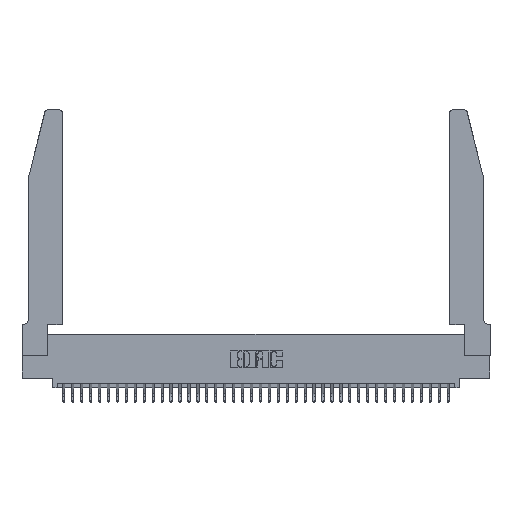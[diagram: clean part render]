
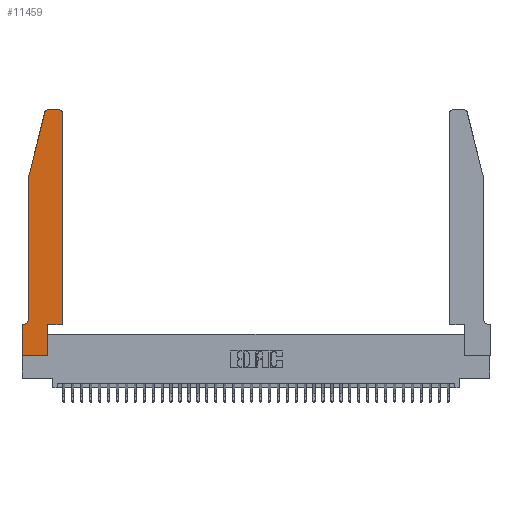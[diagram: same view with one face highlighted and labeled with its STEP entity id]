
A CAD part, top view. The second image highlights one B-rep face of the part: STEP entity #11459.
In plain terms, the highlighted planar face has unit normal (0, 0, 1).
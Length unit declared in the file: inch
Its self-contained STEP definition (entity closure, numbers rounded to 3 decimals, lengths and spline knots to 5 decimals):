
#337 = DIRECTION ( 'NONE',  ( 0., 1., 0. ) ) ;
#662 = CARTESIAN_POINT ( 'NONE',  ( 0.2865, 0.35, 0.37 ) ) ;
#986 = VECTOR ( 'NONE', #16394, 39.37008 ) ;
#1075 = VECTOR ( 'NONE', #16788, 39.37008 ) ;
#1171 = CIRCLE ( 'NONE', #2371, 0.07 ) ;
#1643 = VERTEX_POINT ( 'NONE', #33704 ) ;
#1840 = EDGE_CURVE ( 'NONE', #24150, #3727, #38521, .T. ) ;
#2062 = LINE ( 'NONE', #37913, #1075 ) ;
#2216 = VECTOR ( 'NONE', #2494, 39.37008 ) ;
#2371 = AXIS2_PLACEMENT_3D ( 'NONE', #33833, #15726, #36857 ) ;
#2494 = DIRECTION ( 'NONE',  ( 1., 0., 0. ) ) ;
#3075 = CARTESIAN_POINT ( 'NONE',  ( 0.4505, 0.35, 0.37 ) ) ;
#3687 = ORIENTED_EDGE ( 'NONE', *, *, #26643, .T. ) ;
#3727 = VERTEX_POINT ( 'NONE', #38677 ) ;
#3834 = CARTESIAN_POINT ( 'NONE',  ( 0.0755, 0.35, 0.37 ) ) ;
#4285 = VERTEX_POINT ( 'NONE', #16889 ) ;
#4536 = VERTEX_POINT ( 'NONE', #33355 ) ;
#5559 = AXIS2_PLACEMENT_3D ( 'NONE', #28609, #31632, #13505 ) ;
#5851 = ORIENTED_EDGE ( 'NONE', *, *, #1840, .T. ) ;
#5987 = ORIENTED_EDGE ( 'NONE', *, *, #37012, .T. ) ;
#7193 = VECTOR ( 'NONE', #27434, 39.37008 ) ;
#7437 = PLANE ( 'NONE',  #5559 ) ;
#7518 = VERTEX_POINT ( 'NONE', #23791 ) ;
#7654 = EDGE_CURVE ( 'NONE', #15623, #4536, #24284, .T. ) ;
#7711 = EDGE_CURVE ( 'NONE', #11167, #20975, #37471, .T. ) ;
#7770 = DIRECTION ( 'NONE',  ( 1., 0., 0. ) ) ;
#8392 = EDGE_CURVE ( 'NONE', #1643, #7518, #29853, .T. ) ;
#8755 = ORIENTED_EDGE ( 'NONE', *, *, #18602, .T. ) ;
#9284 = CARTESIAN_POINT ( 'NONE',  ( 0.2605, 2.75, 0.37 ) ) ;
#9593 = LINE ( 'NONE', #31826, #16731 ) ;
#10157 = EDGE_CURVE ( 'NONE', #13219, #1643, #2062, .T. ) ;
#10722 = CARTESIAN_POINT ( 'NONE',  ( 0.25487, 2.72718, 0.37 ) ) ;
#11167 = VERTEX_POINT ( 'NONE', #3075 ) ;
#11459 = ADVANCED_FACE ( 'NONE', ( #19196 ), #7437, .T. ) ;
#11560 = CARTESIAN_POINT ( 'NONE',  ( 0.0055, 0.35, 0.37 ) ) ;
#13219 = VERTEX_POINT ( 'NONE', #10722 ) ;
#13344 = VECTOR ( 'NONE', #337, 39.37008 ) ;
#13505 = DIRECTION ( 'NONE',  ( 1., 0., 0. ) ) ;
#15623 = VERTEX_POINT ( 'NONE', #29559 ) ;
#15726 = DIRECTION ( 'NONE',  ( 0., 0., -1. ) ) ;
#16394 = DIRECTION ( 'NONE',  ( 0., -1., 0. ) ) ;
#16698 = ORIENTED_EDGE ( 'NONE', *, *, #8392, .T. ) ;
#16731 = VECTOR ( 'NONE', #7770, 39.37008 ) ;
#16788 = DIRECTION ( 'NONE',  ( -0.239, -0.971, 0. ) ) ;
#16808 = CARTESIAN_POINT ( 'NONE',  ( 0.4205, 2.72, 0.37 ) ) ;
#16889 = CARTESIAN_POINT ( 'NONE',  ( 0.2865, 0., 0.37 ) ) ;
#17036 = EDGE_CURVE ( 'NONE', #31985, #24150, #18459, .T. ) ;
#17488 = CIRCLE ( 'NONE', #30842, 0.03 ) ;
#17507 = VECTOR ( 'NONE', #19046, 39.37008 ) ;
#18123 = DIRECTION ( 'NONE',  ( 0., 0., 1. ) ) ;
#18459 = LINE ( 'NONE', #3834, #17507 ) ;
#18602 = EDGE_CURVE ( 'NONE', #20975, #15623, #19787, .T. ) ;
#19046 = DIRECTION ( 'NONE',  ( -1., 0., 0. ) ) ;
#19059 = VECTOR ( 'NONE', #31043, 39.37008 ) ;
#19196 = FACE_OUTER_BOUND ( 'NONE', #32320, .T. ) ;
#19377 = ORIENTED_EDGE ( 'NONE', *, *, #10157, .T. ) ;
#19787 = CIRCLE ( 'NONE', #26524, 0.03 ) ;
#19893 = DIRECTION ( 'NONE',  ( 1., 0., 0. ) ) ;
#20975 = VERTEX_POINT ( 'NONE', #24878 ) ;
#22648 = EDGE_CURVE ( 'NONE', #7518, #31985, #1171, .T. ) ;
#22881 = ORIENTED_EDGE ( 'NONE', *, *, #28454, .T. ) ;
#23595 = VERTEX_POINT ( 'NONE', #32441 ) ;
#23791 = CARTESIAN_POINT ( 'NONE',  ( 0.0755, 0.42, 0.37 ) ) ;
#24150 = VERTEX_POINT ( 'NONE', #37436 ) ;
#24284 = LINE ( 'NONE', #9284, #7193 ) ;
#24878 = CARTESIAN_POINT ( 'NONE',  ( 0.4505, 2.72, 0.37 ) ) ;
#26523 = LINE ( 'NONE', #38812, #2216 ) ;
#26524 = AXIS2_PLACEMENT_3D ( 'NONE', #16808, #37927, #19893 ) ;
#26643 = EDGE_CURVE ( 'NONE', #4285, #23595, #35087, .T. ) ;
#27434 = DIRECTION ( 'NONE',  ( -1., 0., 0. ) ) ;
#27994 = ORIENTED_EDGE ( 'NONE', *, *, #22648, .T. ) ;
#28454 = EDGE_CURVE ( 'NONE', #23595, #11167, #26523, .T. ) ;
#28609 = CARTESIAN_POINT ( 'NONE',  ( 0., 0.35, 0.37 ) ) ;
#28737 = ORIENTED_EDGE ( 'NONE', *, *, #7654, .T. ) ;
#29559 = CARTESIAN_POINT ( 'NONE',  ( 0.4205, 2.75, 0.37 ) ) ;
#29853 = LINE ( 'NONE', #34240, #36913 ) ;
#30340 = ORIENTED_EDGE ( 'NONE', *, *, #31391, .T. ) ;
#30842 = AXIS2_PLACEMENT_3D ( 'NONE', #36177, #18123, #39199 ) ;
#31043 = DIRECTION ( 'NONE',  ( 0., 1., 0. ) ) ;
#31226 = DIRECTION ( 'NONE',  ( 0., -1., 0. ) ) ;
#31391 = EDGE_CURVE ( 'NONE', #4536, #13219, #17488, .T. ) ;
#31464 = CARTESIAN_POINT ( 'NONE',  ( 0., 0., 0.37 ) ) ;
#31632 = DIRECTION ( 'NONE',  ( 0., 0., 1. ) ) ;
#31826 = CARTESIAN_POINT ( 'NONE',  ( 0., 0., 0.37 ) ) ;
#31985 = VERTEX_POINT ( 'NONE', #11560 ) ;
#32320 = EDGE_LOOP ( 'NONE', ( #28737, #30340, #19377, #16698, #27994, #34795, #5851, #5987, #3687, #22881, #36824, #8755 ) ) ;
#32441 = CARTESIAN_POINT ( 'NONE',  ( 0.2865, 0.35, 0.37 ) ) ;
#33355 = CARTESIAN_POINT ( 'NONE',  ( 0.284, 2.75, 0.37 ) ) ;
#33704 = CARTESIAN_POINT ( 'NONE',  ( 0.0755, 2., 0.37 ) ) ;
#33833 = CARTESIAN_POINT ( 'NONE',  ( 0.0055, 0.42, 0.37 ) ) ;
#34240 = CARTESIAN_POINT ( 'NONE',  ( 0.0755, 2., 0.37 ) ) ;
#34795 = ORIENTED_EDGE ( 'NONE', *, *, #17036, .T. ) ;
#35087 = LINE ( 'NONE', #662, #19059 ) ;
#36177 = CARTESIAN_POINT ( 'NONE',  ( 0.284, 2.72, 0.37 ) ) ;
#36788 = CARTESIAN_POINT ( 'NONE',  ( 0.4505, 0.35, 0.37 ) ) ;
#36824 = ORIENTED_EDGE ( 'NONE', *, *, #7711, .T. ) ;
#36857 = DIRECTION ( 'NONE',  ( -1., 0., 0. ) ) ;
#36913 = VECTOR ( 'NONE', #31226, 39.37008 ) ;
#37012 = EDGE_CURVE ( 'NONE', #3727, #4285, #9593, .T. ) ;
#37436 = CARTESIAN_POINT ( 'NONE',  ( 0., 0.35, 0.37 ) ) ;
#37471 = LINE ( 'NONE', #36788, #13344 ) ;
#37913 = CARTESIAN_POINT ( 'NONE',  ( 0.0755, 2., 0.37 ) ) ;
#37927 = DIRECTION ( 'NONE',  ( 0., 0., 1. ) ) ;
#38521 = LINE ( 'NONE', #31464, #986 ) ;
#38677 = CARTESIAN_POINT ( 'NONE',  ( 0., 0., 0.37 ) ) ;
#38812 = CARTESIAN_POINT ( 'NONE',  ( 0.4505, 0.35, 0.37 ) ) ;
#39199 = DIRECTION ( 'NONE',  ( 1., 0., 0. ) ) ;
